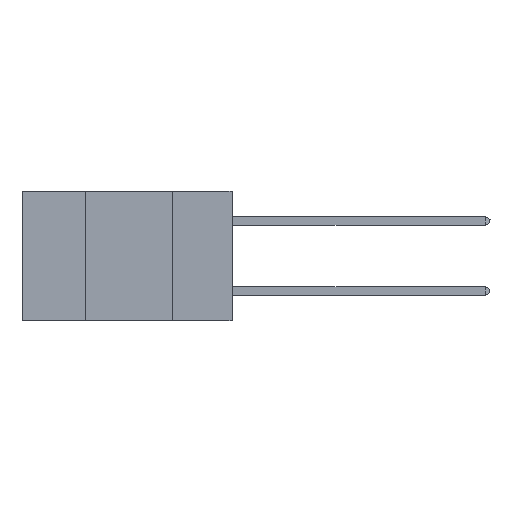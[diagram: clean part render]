
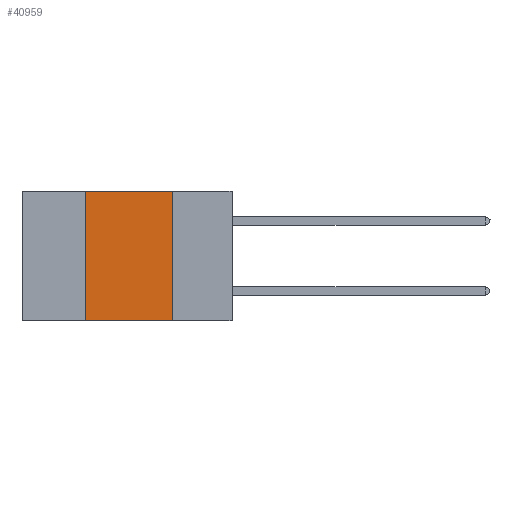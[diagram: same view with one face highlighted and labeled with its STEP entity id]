
A CAD part, left-side view. The second image highlights one B-rep face of the part: STEP entity #40959.
In plain terms, the highlighted planar face has unit normal (-1, 0, 0).
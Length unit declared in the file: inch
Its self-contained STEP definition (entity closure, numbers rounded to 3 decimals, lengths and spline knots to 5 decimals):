
#455 = VERTEX_POINT ( 'NONE', #12495 ) ;
#4444 = CARTESIAN_POINT ( 'NONE',  ( 0., 0.42, 0. ) ) ;
#6063 = DIRECTION ( 'NONE',  ( 0., 0., -1. ) ) ;
#6922 = ORIENTED_EDGE ( 'NONE', *, *, #22260, .F. ) ;
#7334 = EDGE_CURVE ( 'NONE', #18007, #38662, #28145, .T. ) ;
#7453 = EDGE_LOOP ( 'NONE', ( #15462, #41786, #6922, #25098 ) ) ;
#9631 = VERTEX_POINT ( 'NONE', #4444 ) ;
#12495 = CARTESIAN_POINT ( 'NONE',  ( 0., 0.17, 0. ) ) ;
#15462 = ORIENTED_EDGE ( 'NONE', *, *, #20976, .F. ) ;
#16537 = VECTOR ( 'NONE', #17472, 39.37008 ) ;
#17289 = LINE ( 'NONE', #32166, #41204 ) ;
#17472 = DIRECTION ( 'NONE',  ( 0., 0., -1. ) ) ;
#18007 = VERTEX_POINT ( 'NONE', #24048 ) ;
#20976 = EDGE_CURVE ( 'NONE', #455, #38662, #40275, .T. ) ;
#21049 = LINE ( 'NONE', #43374, #34094 ) ;
#22260 = EDGE_CURVE ( 'NONE', #18007, #9631, #17289, .T. ) ;
#24048 = CARTESIAN_POINT ( 'NONE',  ( 0., 0.42, -0.37 ) ) ;
#24377 = EDGE_CURVE ( 'NONE', #9631, #455, #21049, .T. ) ;
#24647 = DIRECTION ( 'NONE',  ( 1., 0., 0. ) ) ;
#25098 = ORIENTED_EDGE ( 'NONE', *, *, #7334, .T. ) ;
#28145 = LINE ( 'NONE', #43272, #31535 ) ;
#31535 = VECTOR ( 'NONE', #35832, 39.37008 ) ;
#32166 = CARTESIAN_POINT ( 'NONE',  ( 0., 0.42, 0. ) ) ;
#32317 = FACE_OUTER_BOUND ( 'NONE', #7453, .T. ) ;
#34094 = VECTOR ( 'NONE', #35689, 39.37008 ) ;
#35689 = DIRECTION ( 'NONE',  ( 0., -1., 0. ) ) ;
#35832 = DIRECTION ( 'NONE',  ( 0., -1., 0. ) ) ;
#38662 = VERTEX_POINT ( 'NONE', #40418 ) ;
#39007 = AXIS2_PLACEMENT_3D ( 'NONE', #40004, #24647, #6063 ) ;
#40004 = CARTESIAN_POINT ( 'NONE',  ( 0., 0.6, 0. ) ) ;
#40275 = LINE ( 'NONE', #47230, #16537 ) ;
#40418 = CARTESIAN_POINT ( 'NONE',  ( 0., 0.17, -0.37 ) ) ;
#40959 = ADVANCED_FACE ( 'NONE', ( #32317 ), #43731, .F. ) ;
#41204 = VECTOR ( 'NONE', #47305, 39.37008 ) ;
#41786 = ORIENTED_EDGE ( 'NONE', *, *, #24377, .F. ) ;
#43272 = CARTESIAN_POINT ( 'NONE',  ( 0., 0.6, -0.37 ) ) ;
#43374 = CARTESIAN_POINT ( 'NONE',  ( 0., 0.6, 0. ) ) ;
#43731 = PLANE ( 'NONE',  #39007 ) ;
#47230 = CARTESIAN_POINT ( 'NONE',  ( 0., 0.17, 0. ) ) ;
#47305 = DIRECTION ( 'NONE',  ( 0., 0., 1. ) ) ;
